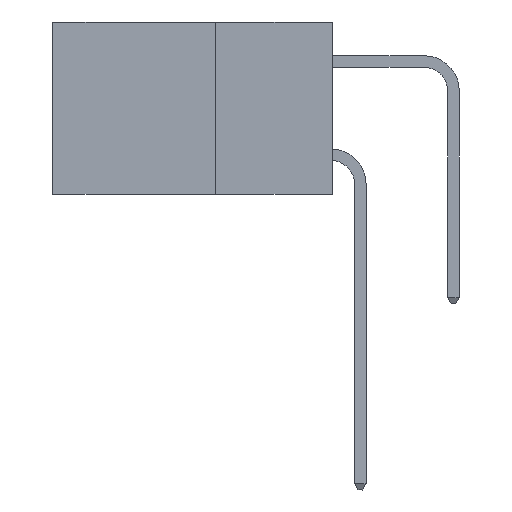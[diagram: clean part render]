
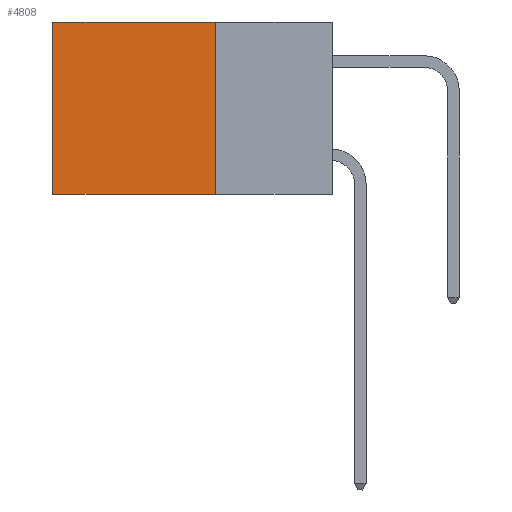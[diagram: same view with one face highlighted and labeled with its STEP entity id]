
A CAD part, left-side view. The second image highlights one B-rep face of the part: STEP entity #4808.
In plain terms, the highlighted planar face has unit normal (-1, 0, 0).
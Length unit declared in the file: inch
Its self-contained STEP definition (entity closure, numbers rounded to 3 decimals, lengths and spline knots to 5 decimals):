
#572 = EDGE_CURVE ( 'NONE', #793, #1397, #6436, .T. ) ;
#793 = VERTEX_POINT ( 'NONE', #3407 ) ;
#1027 = VECTOR ( 'NONE', #10057, 39.37008 ) ;
#1219 = VERTEX_POINT ( 'NONE', #8454 ) ;
#1239 = EDGE_CURVE ( 'NONE', #793, #3411, #6295, .T. ) ;
#1397 = VERTEX_POINT ( 'NONE', #8266 ) ;
#1730 = EDGE_CURVE ( 'NONE', #1397, #1219, #3224, .T. ) ;
#3224 = LINE ( 'NONE', #8816, #1027 ) ;
#3356 = EDGE_LOOP ( 'NONE', ( #5736, #9726, #11001, #6767 ) ) ;
#3407 = CARTESIAN_POINT ( 'NONE',  ( 0.298, 0.25, 0. ) ) ;
#3411 = VERTEX_POINT ( 'NONE', #6330 ) ;
#3985 = CARTESIAN_POINT ( 'NONE',  ( 0.298, 0.25, 0. ) ) ;
#3989 = EDGE_CURVE ( 'NONE', #3411, #1219, #9417, .T. ) ;
#4126 = DIRECTION ( 'NONE',  ( 0., 0., -1. ) ) ;
#4182 = VECTOR ( 'NONE', #5594, 39.37008 ) ;
#4711 = VECTOR ( 'NONE', #4126, 39.37008 ) ;
#4808 = ADVANCED_FACE ( 'NONE', ( #9955 ), #10107, .F. ) ;
#5114 = DIRECTION ( 'NONE',  ( 0., 0., -1. ) ) ;
#5529 = CARTESIAN_POINT ( 'NONE',  ( 0.298, 0.25, 0. ) ) ;
#5594 = DIRECTION ( 'NONE',  ( 0., 0., -1. ) ) ;
#5736 = ORIENTED_EDGE ( 'NONE', *, *, #3989, .T. ) ;
#6295 = LINE ( 'NONE', #10180, #10719 ) ;
#6330 = CARTESIAN_POINT ( 'NONE',  ( 0.298, 0.6, 0. ) ) ;
#6436 = LINE ( 'NONE', #5529, #4182 ) ;
#6767 = ORIENTED_EDGE ( 'NONE', *, *, #1239, .T. ) ;
#8266 = CARTESIAN_POINT ( 'NONE',  ( 0.298, 0.25, -0.37 ) ) ;
#8454 = CARTESIAN_POINT ( 'NONE',  ( 0.298, 0.6, -0.37 ) ) ;
#8467 = CARTESIAN_POINT ( 'NONE',  ( 0.298, 0.6, 0. ) ) ;
#8816 = CARTESIAN_POINT ( 'NONE',  ( 0.298, 0.25, -0.37 ) ) ;
#9417 = LINE ( 'NONE', #8467, #4711 ) ;
#9726 = ORIENTED_EDGE ( 'NONE', *, *, #1730, .F. ) ;
#9807 = AXIS2_PLACEMENT_3D ( 'NONE', #3985, #9878, #5114 ) ;
#9878 = DIRECTION ( 'NONE',  ( 1., 0., 0. ) ) ;
#9955 = FACE_OUTER_BOUND ( 'NONE', #3356, .T. ) ;
#10057 = DIRECTION ( 'NONE',  ( 0., 1., 0. ) ) ;
#10107 = PLANE ( 'NONE',  #9807 ) ;
#10180 = CARTESIAN_POINT ( 'NONE',  ( 0.298, 0.25, 0. ) ) ;
#10719 = VECTOR ( 'NONE', #10944, 39.37008 ) ;
#10944 = DIRECTION ( 'NONE',  ( 0., 1., 0. ) ) ;
#11001 = ORIENTED_EDGE ( 'NONE', *, *, #572, .F. ) ;
